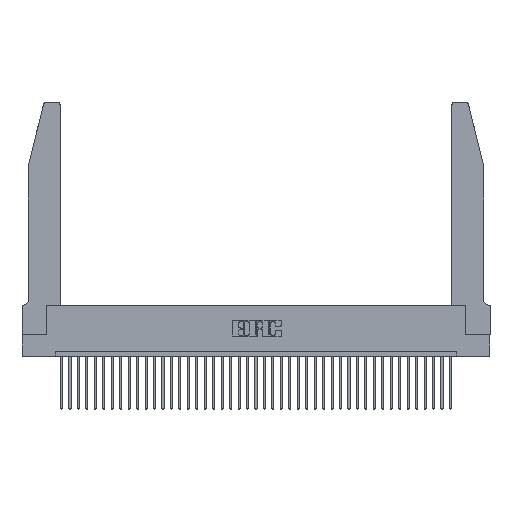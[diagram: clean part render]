
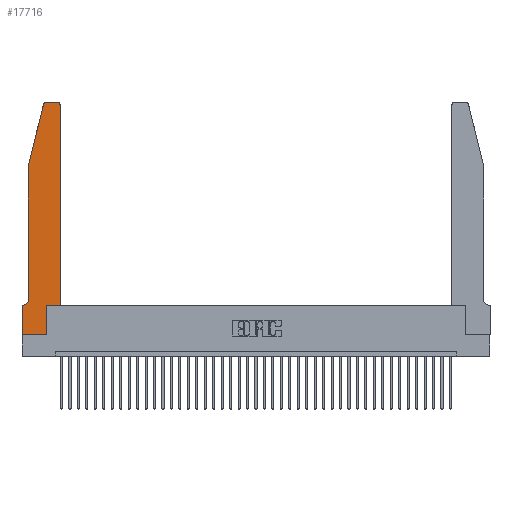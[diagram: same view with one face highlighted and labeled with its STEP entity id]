
A CAD part, top view. The second image highlights one B-rep face of the part: STEP entity #17716.
In plain terms, the highlighted planar face has unit normal (0, 0, 1).
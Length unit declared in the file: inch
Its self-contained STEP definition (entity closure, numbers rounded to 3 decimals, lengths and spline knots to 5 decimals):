
#406 = EDGE_CURVE ( 'NONE', #14215, #14896, #5689, .T. ) ;
#423 = DIRECTION ( 'NONE',  ( 0., 0., 1. ) ) ;
#604 = CARTESIAN_POINT ( 'NONE',  ( 0.25487, 2.72718, 0.37 ) ) ;
#767 = DIRECTION ( 'NONE',  ( -0.239, -0.971, 0. ) ) ;
#1048 = ORIENTED_EDGE ( 'NONE', *, *, #2699, .T. ) ;
#1606 = LINE ( 'NONE', #22000, #15009 ) ;
#1801 = VECTOR ( 'NONE', #21329, 39.37008 ) ;
#1859 = CARTESIAN_POINT ( 'NONE',  ( 0.0755, 0.35, 0.37 ) ) ;
#2407 = CIRCLE ( 'NONE', #17181, 0.03 ) ;
#2567 = DIRECTION ( 'NONE',  ( 1., 0., 0. ) ) ;
#2699 = EDGE_CURVE ( 'NONE', #33006, #17551, #1606, .T. ) ;
#3357 = DIRECTION ( 'NONE',  ( -1., 0., 0. ) ) ;
#4462 = CIRCLE ( 'NONE', #4542, 0.03 ) ;
#4509 = EDGE_CURVE ( 'NONE', #14896, #20571, #4462, .T. ) ;
#4542 = AXIS2_PLACEMENT_3D ( 'NONE', #15701, #423, #21864 ) ;
#5582 = DIRECTION ( 'NONE',  ( 1., 0., 0. ) ) ;
#5689 = LINE ( 'NONE', #33689, #1801 ) ;
#6627 = VECTOR ( 'NONE', #767, 39.37008 ) ;
#6747 = EDGE_CURVE ( 'NONE', #34714, #9302, #12696, .T. ) ;
#7094 = DIRECTION ( 'NONE',  ( -1., 0., 0. ) ) ;
#9302 = VERTEX_POINT ( 'NONE', #16704 ) ;
#9726 = EDGE_CURVE ( 'NONE', #27248, #27444, #2407, .T. ) ;
#10314 = DIRECTION ( 'NONE',  ( 1., 0., 0. ) ) ;
#10382 = AXIS2_PLACEMENT_3D ( 'NONE', #31239, #16015, #7094 ) ;
#11063 = DIRECTION ( 'NONE',  ( 0., -1., 0. ) ) ;
#11084 = CARTESIAN_POINT ( 'NONE',  ( 0.0055, 0.35, 0.37 ) ) ;
#11315 = VERTEX_POINT ( 'NONE', #11084 ) ;
#11532 = DIRECTION ( 'NONE',  ( 0., 1., 0. ) ) ;
#12409 = CARTESIAN_POINT ( 'NONE',  ( 0.0755, 2., 0.37 ) ) ;
#12696 = LINE ( 'NONE', #26587, #16535 ) ;
#13187 = ORIENTED_EDGE ( 'NONE', *, *, #35582, .T. ) ;
#13246 = EDGE_LOOP ( 'NONE', ( #34387, #13789, #20646, #1048, #13187, #22098, #39181, #35712, #20933, #17709, #35704, #14654 ) ) ;
#13789 = ORIENTED_EDGE ( 'NONE', *, *, #9726, .T. ) ;
#13991 = VECTOR ( 'NONE', #3357, 39.37008 ) ;
#14215 = VERTEX_POINT ( 'NONE', #23202 ) ;
#14654 = ORIENTED_EDGE ( 'NONE', *, *, #4509, .T. ) ;
#14896 = VERTEX_POINT ( 'NONE', #36999 ) ;
#15009 = VECTOR ( 'NONE', #22390, 39.37008 ) ;
#15149 = VERTEX_POINT ( 'NONE', #16911 ) ;
#15292 = CARTESIAN_POINT ( 'NONE',  ( 0., 0.35, 0.37 ) ) ;
#15701 = CARTESIAN_POINT ( 'NONE',  ( 0.4205, 2.72, 0.37 ) ) ;
#16015 = DIRECTION ( 'NONE',  ( 0., 0., -1. ) ) ;
#16311 = EDGE_CURVE ( 'NONE', #27444, #33006, #35261, .T. ) ;
#16535 = VECTOR ( 'NONE', #11532, 39.37008 ) ;
#16704 = CARTESIAN_POINT ( 'NONE',  ( 0.2865, 0.35, 0.37 ) ) ;
#16911 = CARTESIAN_POINT ( 'NONE',  ( 0., 0., 0.37 ) ) ;
#17181 = AXIS2_PLACEMENT_3D ( 'NONE', #24226, #27289, #2567 ) ;
#17551 = VERTEX_POINT ( 'NONE', #18497 ) ;
#17709 = ORIENTED_EDGE ( 'NONE', *, *, #18669, .T. ) ;
#17716 = ADVANCED_FACE ( 'NONE', ( #33567 ), #33574, .T. ) ;
#18497 = CARTESIAN_POINT ( 'NONE',  ( 0.0755, 0.42, 0.37 ) ) ;
#18669 = EDGE_CURVE ( 'NONE', #9302, #14215, #35950, .T. ) ;
#18960 = LINE ( 'NONE', #25394, #38489 ) ;
#20260 = VERTEX_POINT ( 'NONE', #38590 ) ;
#20571 = VERTEX_POINT ( 'NONE', #21367 ) ;
#20646 = ORIENTED_EDGE ( 'NONE', *, *, #16311, .T. ) ;
#20933 = ORIENTED_EDGE ( 'NONE', *, *, #6747, .T. ) ;
#21329 = DIRECTION ( 'NONE',  ( 0., 1., 0. ) ) ;
#21367 = CARTESIAN_POINT ( 'NONE',  ( 0.4205, 2.75, 0.37 ) ) ;
#21679 = CARTESIAN_POINT ( 'NONE',  ( 0.2605, 2.75, 0.37 ) ) ;
#21864 = DIRECTION ( 'NONE',  ( 1., 0., 0. ) ) ;
#22000 = CARTESIAN_POINT ( 'NONE',  ( 0.0755, 2., 0.37 ) ) ;
#22098 = ORIENTED_EDGE ( 'NONE', *, *, #37787, .T. ) ;
#22390 = DIRECTION ( 'NONE',  ( 0., -1., 0. ) ) ;
#23202 = CARTESIAN_POINT ( 'NONE',  ( 0.4505, 0.35, 0.37 ) ) ;
#24226 = CARTESIAN_POINT ( 'NONE',  ( 0.284, 2.72, 0.37 ) ) ;
#24482 = EDGE_CURVE ( 'NONE', #20260, #15149, #37095, .T. ) ;
#25229 = DIRECTION ( 'NONE',  ( 1., 0., 0. ) ) ;
#25394 = CARTESIAN_POINT ( 'NONE',  ( 0., 0., 0.37 ) ) ;
#26587 = CARTESIAN_POINT ( 'NONE',  ( 0.2865, 0.35, 0.37 ) ) ;
#26972 = CARTESIAN_POINT ( 'NONE',  ( 0.2865, 0., 0.37 ) ) ;
#27200 = VECTOR ( 'NONE', #11063, 39.37008 ) ;
#27219 = VECTOR ( 'NONE', #32449, 39.37008 ) ;
#27248 = VERTEX_POINT ( 'NONE', #28888 ) ;
#27289 = DIRECTION ( 'NONE',  ( 0., 0., 1. ) ) ;
#27393 = LINE ( 'NONE', #21679, #13991 ) ;
#27444 = VERTEX_POINT ( 'NONE', #604 ) ;
#27448 = CARTESIAN_POINT ( 'NONE',  ( 0.0755, 2., 0.37 ) ) ;
#28467 = EDGE_CURVE ( 'NONE', #20571, #27248, #27393, .T. ) ;
#28888 = CARTESIAN_POINT ( 'NONE',  ( 0.284, 2.75, 0.37 ) ) ;
#30718 = VECTOR ( 'NONE', #25229, 39.37008 ) ;
#31239 = CARTESIAN_POINT ( 'NONE',  ( 0.0055, 0.42, 0.37 ) ) ;
#31540 = CIRCLE ( 'NONE', #10382, 0.07 ) ;
#31734 = EDGE_CURVE ( 'NONE', #15149, #34714, #18960, .T. ) ;
#32449 = DIRECTION ( 'NONE',  ( -1., 0., 0. ) ) ;
#33006 = VERTEX_POINT ( 'NONE', #12409 ) ;
#33075 = DIRECTION ( 'NONE',  ( 0., 0., 1. ) ) ;
#33567 = FACE_OUTER_BOUND ( 'NONE', #13246, .T. ) ;
#33574 = PLANE ( 'NONE',  #34689 ) ;
#33689 = CARTESIAN_POINT ( 'NONE',  ( 0.4505, 0.35, 0.37 ) ) ;
#34387 = ORIENTED_EDGE ( 'NONE', *, *, #28467, .T. ) ;
#34689 = AXIS2_PLACEMENT_3D ( 'NONE', #15292, #33075, #5582 ) ;
#34714 = VERTEX_POINT ( 'NONE', #26972 ) ;
#35261 = LINE ( 'NONE', #27448, #6627 ) ;
#35582 = EDGE_CURVE ( 'NONE', #17551, #11315, #31540, .T. ) ;
#35704 = ORIENTED_EDGE ( 'NONE', *, *, #406, .T. ) ;
#35712 = ORIENTED_EDGE ( 'NONE', *, *, #31734, .T. ) ;
#35950 = LINE ( 'NONE', #37424, #30718 ) ;
#36254 = LINE ( 'NONE', #1859, #27219 ) ;
#36999 = CARTESIAN_POINT ( 'NONE',  ( 0.4505, 2.72, 0.37 ) ) ;
#37095 = LINE ( 'NONE', #38322, #27200 ) ;
#37424 = CARTESIAN_POINT ( 'NONE',  ( 0.4505, 0.35, 0.37 ) ) ;
#37787 = EDGE_CURVE ( 'NONE', #11315, #20260, #36254, .T. ) ;
#38322 = CARTESIAN_POINT ( 'NONE',  ( 0., 0., 0.37 ) ) ;
#38489 = VECTOR ( 'NONE', #10314, 39.37008 ) ;
#38590 = CARTESIAN_POINT ( 'NONE',  ( 0., 0.35, 0.37 ) ) ;
#39181 = ORIENTED_EDGE ( 'NONE', *, *, #24482, .T. ) ;
